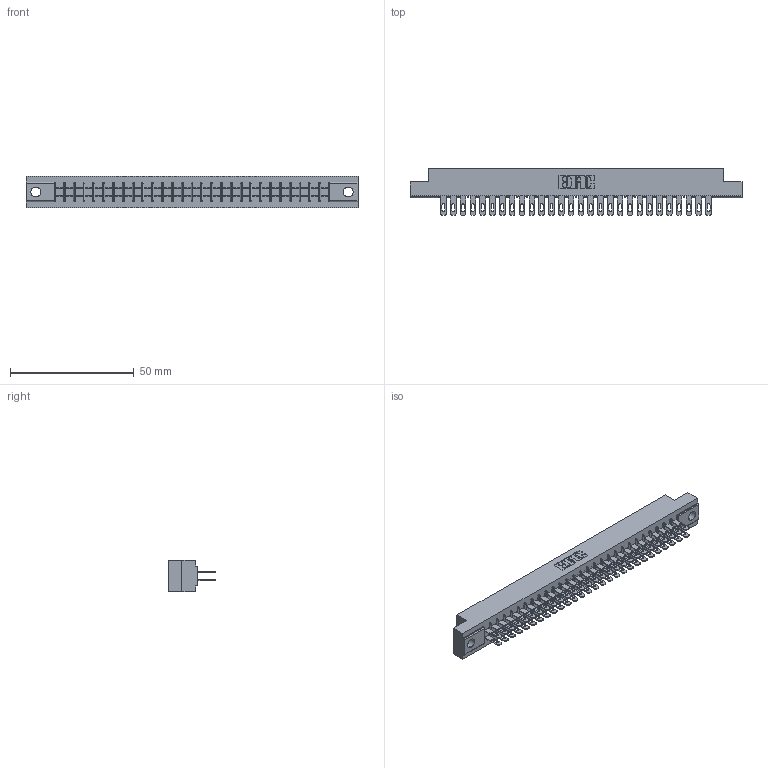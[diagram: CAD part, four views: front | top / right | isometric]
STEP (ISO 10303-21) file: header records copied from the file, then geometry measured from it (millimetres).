
FILE_DESCRIPTION (( 'STEP AP203' ), '1' );
FILE_NAME ('305-056-500-504.STEP', '2019-09-09T23:30:28', ( '' ), ( '' ), 'SwSTEP 2.0', 'SolidWorks 2016', '' );
FILE_SCHEMA (( 'CONFIG_CONTROL_DESIGN' ));
Length unit declared in the file: inch
Products named in the file (3): 305-290-001_500; 305-056-500-504; 305 Part_.156 Dia
Assembly tree (57 placements, depth 2):
  305-056-500-504
    305 Part_.156 Dia
    305-290-001_500  x56
Bounding box: 133.96 x 18.85 x 12.7 mm (x, y, z)
Volume: 13569.8 mm3; surface area: 18501.6 mm2
Topology: 57 solids, 57 shells, 2930 faces, 8388 edges, 5440 vertices
Faces by surface type: plane 1650, cylinder 1168, sphere 112
Entity records: 32461 total; most frequent: CARTESIAN_POINT 5376, ORIENTED_EDGE 5332, DIRECTION 5206, EDGE_CURVE 2666, LINE 2146, VECTOR 2146, VERTEX_POINT 1700, AXIS2_PLACEMENT_3D 1530
